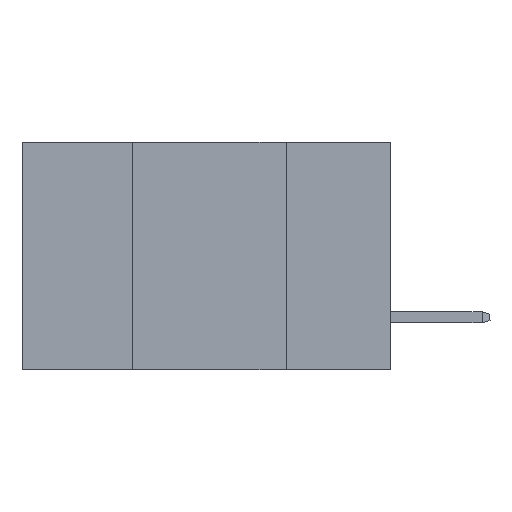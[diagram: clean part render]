
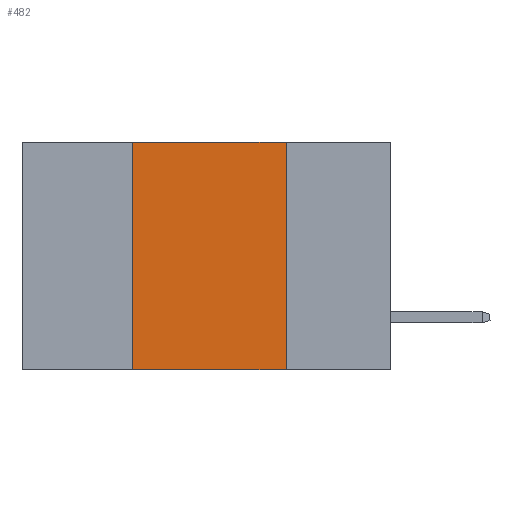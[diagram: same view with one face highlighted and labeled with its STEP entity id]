
A CAD part, left-side view. The second image highlights one B-rep face of the part: STEP entity #482.
In plain terms, the highlighted planar face has unit normal (-1, 0, 0).
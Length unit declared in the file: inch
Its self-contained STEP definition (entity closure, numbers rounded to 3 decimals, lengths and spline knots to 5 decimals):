
#12 = PLANE ( 'NONE',  #2465 ) ;
#299 = LINE ( 'NONE', #896, #16728 ) ;
#482 = ADVANCED_FACE ( 'NONE', ( #843 ), #12, .F. ) ;
#783 = EDGE_LOOP ( 'NONE', ( #19412, #3724, #14050, #7447 ) ) ;
#843 = FACE_OUTER_BOUND ( 'NONE', #783, .T. ) ;
#896 = CARTESIAN_POINT ( 'NONE',  ( 0., 0.6, -0.37 ) ) ;
#1402 = EDGE_CURVE ( 'NONE', #5351, #4134, #299, .T. ) ;
#1574 = DIRECTION ( 'NONE',  ( 0., 0., -1. ) ) ;
#2465 = AXIS2_PLACEMENT_3D ( 'NONE', #7592, #20493, #12139 ) ;
#2855 = VERTEX_POINT ( 'NONE', #17153 ) ;
#3226 = DIRECTION ( 'NONE',  ( 0., -1., 0. ) ) ;
#3724 = ORIENTED_EDGE ( 'NONE', *, *, #8397, .F. ) ;
#4134 = VERTEX_POINT ( 'NONE', #13847 ) ;
#5351 = VERTEX_POINT ( 'NONE', #18231 ) ;
#5389 = CARTESIAN_POINT ( 'NONE',  ( 0., 0.42, 0. ) ) ;
#5762 = LINE ( 'NONE', #9604, #14635 ) ;
#6649 = EDGE_CURVE ( 'NONE', #5351, #15182, #8251, .T. ) ;
#7447 = ORIENTED_EDGE ( 'NONE', *, *, #1402, .T. ) ;
#7592 = CARTESIAN_POINT ( 'NONE',  ( 0., 0.6, 0. ) ) ;
#8163 = LINE ( 'NONE', #17427, #16041 ) ;
#8251 = LINE ( 'NONE', #16730, #16619 ) ;
#8397 = EDGE_CURVE ( 'NONE', #15182, #2855, #8163, .T. ) ;
#9051 = EDGE_CURVE ( 'NONE', #2855, #4134, #5762, .T. ) ;
#9604 = CARTESIAN_POINT ( 'NONE',  ( 0., 0.17, 0. ) ) ;
#12139 = DIRECTION ( 'NONE',  ( 0., 0., -1. ) ) ;
#13518 = DIRECTION ( 'NONE',  ( 0., 0., 1. ) ) ;
#13847 = CARTESIAN_POINT ( 'NONE',  ( 0., 0.17, -0.37 ) ) ;
#14050 = ORIENTED_EDGE ( 'NONE', *, *, #6649, .F. ) ;
#14635 = VECTOR ( 'NONE', #1574, 39.37008 ) ;
#15182 = VERTEX_POINT ( 'NONE', #5389 ) ;
#16041 = VECTOR ( 'NONE', #3226, 39.37008 ) ;
#16075 = DIRECTION ( 'NONE',  ( 0., -1., 0. ) ) ;
#16619 = VECTOR ( 'NONE', #13518, 39.37008 ) ;
#16728 = VECTOR ( 'NONE', #16075, 39.37008 ) ;
#16730 = CARTESIAN_POINT ( 'NONE',  ( 0., 0.42, 0. ) ) ;
#17153 = CARTESIAN_POINT ( 'NONE',  ( 0., 0.17, 0. ) ) ;
#17427 = CARTESIAN_POINT ( 'NONE',  ( 0., 0.6, 0. ) ) ;
#18231 = CARTESIAN_POINT ( 'NONE',  ( 0., 0.42, -0.37 ) ) ;
#19412 = ORIENTED_EDGE ( 'NONE', *, *, #9051, .F. ) ;
#20493 = DIRECTION ( 'NONE',  ( 1., 0., 0. ) ) ;
